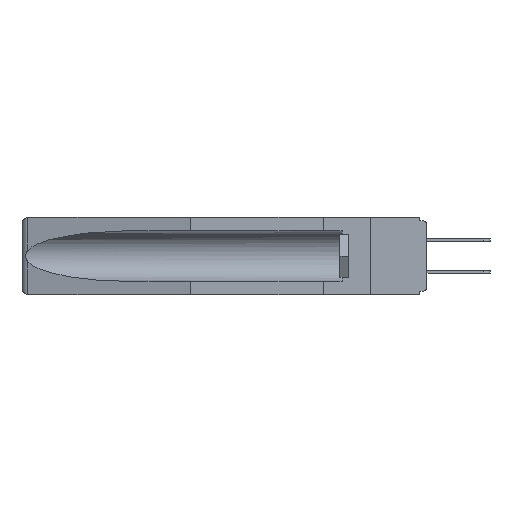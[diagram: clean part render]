
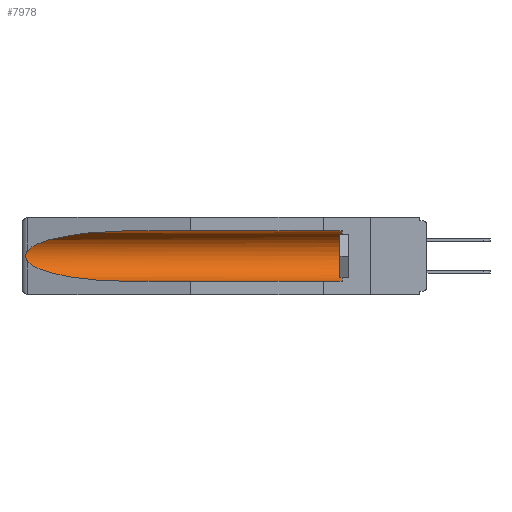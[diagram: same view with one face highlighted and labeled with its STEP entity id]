
A CAD part, left-side view. The second image highlights one B-rep face of the part: STEP entity #7978.
In plain terms, the highlighted cylindrical face has radius 2.857 mm (diameter 5.715 mm), a partial arc.
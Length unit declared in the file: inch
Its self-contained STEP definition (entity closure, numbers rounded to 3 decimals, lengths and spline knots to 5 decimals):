
#579 = DIRECTION ( 'NONE',  ( 0., 1., 0. ) ) ;
#1306 = VECTOR ( 'NONE', #579, 39.37008 ) ;
#1601 = EDGE_CURVE ( 'NONE', #18731, #21103, #4400, .T. ) ;
#1905 = VERTEX_POINT ( 'NONE', #17705 ) ;
#2002 = DIRECTION ( 'NONE',  ( 0., 0., 1. ) ) ;
#2080 = CARTESIAN_POINT ( 'NONE',  ( 0.155, 0.126, -0.1715 ) ) ;
#3726 = EDGE_CURVE ( 'NONE', #15565, #18731, #19073, .T. ) ;
#4400 =( BOUNDED_CURVE ( )  B_SPLINE_CURVE ( 3, ( #15552, #10033, #23013, #17566 ),
 .UNSPECIFIED., .F., .F. ) 
 B_SPLINE_CURVE_WITH_KNOTS ( ( 4, 4 ),
 ( 4.71239, 6.08839 ),
 .UNSPECIFIED. ) 
 CURVE ( )  GEOMETRIC_REPRESENTATION_ITEM ( )  RATIONAL_B_SPLINE_CURVE ( ( 1., 0.848, 0.848, 1. ) ) 
 REPRESENTATION_ITEM ( '' )  );
#4883 = CARTESIAN_POINT ( 'NONE',  ( 0.2675, 1.53308, -0.16763 ) ) ;
#5054 = CARTESIAN_POINT ( 'NONE',  ( 0.2675, 1.53308, -0.17534 ) ) ;
#5553 = CARTESIAN_POINT ( 'NONE',  ( 0.21114, 1.30732, -0.284 ) ) ;
#5809 = CARTESIAN_POINT ( 'NONE',  ( 0.155, -0.30754, -0.284 ) ) ;
#6462 = CARTESIAN_POINT ( 'NONE',  ( 0.26537, 1.52718, -0.14972 ) ) ;
#6480 = B_SPLINE_CURVE_WITH_KNOTS ( 'NONE', 3,
 ( #8885, #21453, #21711, #6841, #4883, #5054, #10436, #12521, #17811, #10353 ),
 .UNSPECIFIED., .F., .F.,
 ( 4, 2, 2, 2, 4 ),
 ( 0., 0.00029, 0.00058, 0.00087, 0.00117 ),
 .UNSPECIFIED. ) ;
#6841 = CARTESIAN_POINT ( 'NONE',  ( 0.2673, 1.5327, -0.16383 ) ) ;
#7260 = EDGE_LOOP ( 'NONE', ( #17586, #22500, #18986, #7281, #11833, #13975 ) ) ;
#7281 = ORIENTED_EDGE ( 'NONE', *, *, #19189, .F. ) ;
#7623 = EDGE_CURVE ( 'NONE', #1905, #9226, #19790, .T. ) ;
#7978 = ADVANCED_FACE ( 'NONE', ( #13142 ), #17448, .F. ) ;
#8134 = VECTOR ( 'NONE', #10786, 39.37008 ) ;
#8258 = LINE ( 'NONE', #5809, #1306 ) ;
#8831 = CARTESIAN_POINT ( 'NONE',  ( 0.155, -0.30754, -0.059 ) ) ;
#8885 = CARTESIAN_POINT ( 'NONE',  ( 0.26537, 1.52718, -0.14972 ) ) ;
#9226 = VERTEX_POINT ( 'NONE', #9911 ) ;
#9274 = DIRECTION ( 'NONE',  ( 0., -1., 0. ) ) ;
#9497 = CARTESIAN_POINT ( 'NONE',  ( 0.155, 1.07973, -0.284 ) ) ;
#9911 = CARTESIAN_POINT ( 'NONE',  ( 0.155, 1.07973, -0.284 ) ) ;
#10033 = CARTESIAN_POINT ( 'NONE',  ( 0.21114, 1.30732, -0.059 ) ) ;
#10353 = CARTESIAN_POINT ( 'NONE',  ( 0.26537, 1.52718, -0.19328 ) ) ;
#10436 = CARTESIAN_POINT ( 'NONE',  ( 0.2673, 1.53269, -0.17917 ) ) ;
#10786 = DIRECTION ( 'NONE',  ( 0., 1., 0. ) ) ;
#10839 = DIRECTION ( 'NONE',  ( 0., 1., 0. ) ) ;
#10917 = VERTEX_POINT ( 'NONE', #12165 ) ;
#11833 = ORIENTED_EDGE ( 'NONE', *, *, #14224, .T. ) ;
#12165 = CARTESIAN_POINT ( 'NONE',  ( 0.155, 0.126, -0.284 ) ) ;
#12521 = CARTESIAN_POINT ( 'NONE',  ( 0.26655, 1.53094, -0.18657 ) ) ;
#13142 = FACE_OUTER_BOUND ( 'NONE', #7260, .T. ) ;
#13975 = ORIENTED_EDGE ( 'NONE', *, *, #3726, .T. ) ;
#14036 = CARTESIAN_POINT ( 'NONE',  ( 0.155, 1.07973, -0.059 ) ) ;
#14224 = EDGE_CURVE ( 'NONE', #10917, #15565, #22751, .T. ) ;
#15552 = CARTESIAN_POINT ( 'NONE',  ( 0.155, 1.07973, -0.059 ) ) ;
#15565 = VERTEX_POINT ( 'NONE', #21480 ) ;
#15599 = AXIS2_PLACEMENT_3D ( 'NONE', #21946, #10839, #18295 ) ;
#16289 = EDGE_CURVE ( 'NONE', #21103, #1905, #6480, .T. ) ;
#16593 = AXIS2_PLACEMENT_3D ( 'NONE', #2080, #9274, #2002 ) ;
#17448 = CYLINDRICAL_SURFACE ( 'NONE', #15599, 0.1125 ) ;
#17566 = CARTESIAN_POINT ( 'NONE',  ( 0.26537, 1.52718, -0.14972 ) ) ;
#17586 = ORIENTED_EDGE ( 'NONE', *, *, #1601, .T. ) ;
#17705 = CARTESIAN_POINT ( 'NONE',  ( 0.26537, 1.52718, -0.19328 ) ) ;
#17811 = CARTESIAN_POINT ( 'NONE',  ( 0.26597, 1.5296, -0.19026 ) ) ;
#18295 = DIRECTION ( 'NONE',  ( 0., 0., 1. ) ) ;
#18558 = CARTESIAN_POINT ( 'NONE',  ( 0.26537, 1.52718, -0.19328 ) ) ;
#18731 = VERTEX_POINT ( 'NONE', #14036 ) ;
#18785 = CARTESIAN_POINT ( 'NONE',  ( 0.25451, 1.48313, -0.24835 ) ) ;
#18986 = ORIENTED_EDGE ( 'NONE', *, *, #7623, .T. ) ;
#19073 = LINE ( 'NONE', #8831, #8134 ) ;
#19189 = EDGE_CURVE ( 'NONE', #10917, #9226, #8258, .T. ) ;
#19790 =( BOUNDED_CURVE ( )  B_SPLINE_CURVE ( 3, ( #18558, #18785, #5553, #9497 ),
 .UNSPECIFIED., .F., .F. ) 
 B_SPLINE_CURVE_WITH_KNOTS ( ( 4, 4 ),
 ( 0.1948, 1.5708 ),
 .UNSPECIFIED. ) 
 CURVE ( )  GEOMETRIC_REPRESENTATION_ITEM ( )  RATIONAL_B_SPLINE_CURVE ( ( 1., 0.848, 0.848, 1. ) ) 
 REPRESENTATION_ITEM ( '' )  );
#21103 = VERTEX_POINT ( 'NONE', #6462 ) ;
#21453 = CARTESIAN_POINT ( 'NONE',  ( 0.26597, 1.52961, -0.15275 ) ) ;
#21480 = CARTESIAN_POINT ( 'NONE',  ( 0.155, 0.126, -0.059 ) ) ;
#21711 = CARTESIAN_POINT ( 'NONE',  ( 0.26654, 1.53092, -0.15636 ) ) ;
#21946 = CARTESIAN_POINT ( 'NONE',  ( 0.155, -0.30754, -0.1715 ) ) ;
#22500 = ORIENTED_EDGE ( 'NONE', *, *, #16289, .T. ) ;
#22751 = CIRCLE ( 'NONE', #16593, 0.1125 ) ;
#23013 = CARTESIAN_POINT ( 'NONE',  ( 0.25451, 1.48313, -0.09465 ) ) ;
